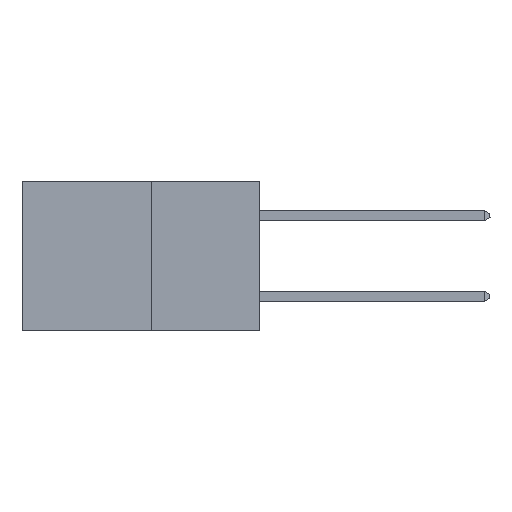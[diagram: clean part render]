
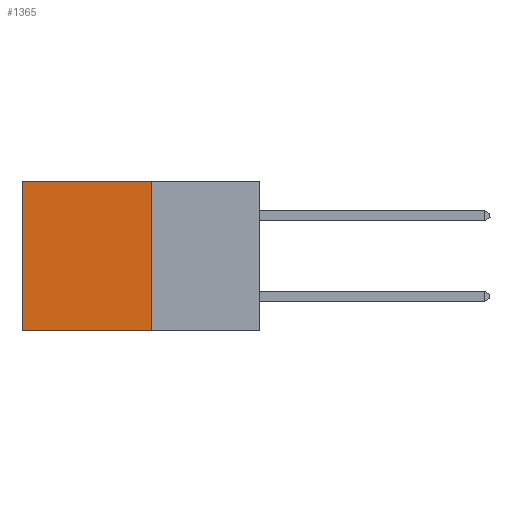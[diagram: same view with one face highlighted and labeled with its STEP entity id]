
A CAD part, left-side view. The second image highlights one B-rep face of the part: STEP entity #1365.
In plain terms, the highlighted planar face has unit normal (-1, 0, 0).
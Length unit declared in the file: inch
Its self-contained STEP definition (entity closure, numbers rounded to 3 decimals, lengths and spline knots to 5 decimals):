
#72 = EDGE_CURVE ( 'NONE', #12732, #971, #12079, .T. ) ;
#971 = VERTEX_POINT ( 'NONE', #7240 ) ;
#1365 = ADVANCED_FACE ( 'NONE', ( #10352 ), #4882, .F. ) ;
#2112 = EDGE_CURVE ( 'NONE', #16244, #12732, #8771, .T. ) ;
#2491 = ORIENTED_EDGE ( 'NONE', *, *, #5827, .F. ) ;
#3877 = VECTOR ( 'NONE', #14639, 39.37008 ) ;
#4882 = PLANE ( 'NONE',  #19514 ) ;
#5083 = CARTESIAN_POINT ( 'NONE',  ( 0.277, 0.59, 0. ) ) ;
#5406 = DIRECTION ( 'NONE',  ( 1., 0., 0. ) ) ;
#5827 = EDGE_CURVE ( 'NONE', #16244, #17717, #15740, .T. ) ;
#6088 = VECTOR ( 'NONE', #16671, 39.37008 ) ;
#6723 = ORIENTED_EDGE ( 'NONE', *, *, #2112, .T. ) ;
#6918 = DIRECTION ( 'NONE',  ( 0., 0., -1. ) ) ;
#7240 = CARTESIAN_POINT ( 'NONE',  ( 0.277, 0.59, -0.37 ) ) ;
#7446 = DIRECTION ( 'NONE',  ( 0., 0., -1. ) ) ;
#7618 = CARTESIAN_POINT ( 'NONE',  ( 0.277, 0.59, -0.37 ) ) ;
#8565 = EDGE_CURVE ( 'NONE', #17717, #971, #8808, .T. ) ;
#8771 = LINE ( 'NONE', #20213, #6088 ) ;
#8808 = LINE ( 'NONE', #16628, #3877 ) ;
#9876 = ORIENTED_EDGE ( 'NONE', *, *, #8565, .F. ) ;
#10352 = FACE_OUTER_BOUND ( 'NONE', #13102, .T. ) ;
#11012 = VECTOR ( 'NONE', #15985, 39.37008 ) ;
#12079 = LINE ( 'NONE', #7618, #15851 ) ;
#12732 = VERTEX_POINT ( 'NONE', #5083 ) ;
#13102 = EDGE_LOOP ( 'NONE', ( #19497, #9876, #2491, #6723 ) ) ;
#13620 = CARTESIAN_POINT ( 'NONE',  ( 0.277, 0.27, -0.37 ) ) ;
#14639 = DIRECTION ( 'NONE',  ( 0., 1., 0. ) ) ;
#15227 = CARTESIAN_POINT ( 'NONE',  ( 0.277, 0.27, -0.37 ) ) ;
#15740 = LINE ( 'NONE', #15227, #11012 ) ;
#15851 = VECTOR ( 'NONE', #7446, 39.37008 ) ;
#15985 = DIRECTION ( 'NONE',  ( 0., 0., -1. ) ) ;
#16244 = VERTEX_POINT ( 'NONE', #19821 ) ;
#16628 = CARTESIAN_POINT ( 'NONE',  ( 0.277, 0.27, -0.37 ) ) ;
#16671 = DIRECTION ( 'NONE',  ( 0., 1., 0. ) ) ;
#17717 = VERTEX_POINT ( 'NONE', #21259 ) ;
#19497 = ORIENTED_EDGE ( 'NONE', *, *, #72, .T. ) ;
#19514 = AXIS2_PLACEMENT_3D ( 'NONE', #13620, #5406, #6918 ) ;
#19821 = CARTESIAN_POINT ( 'NONE',  ( 0.277, 0.27, 0. ) ) ;
#20213 = CARTESIAN_POINT ( 'NONE',  ( 0.277, 0.27, 0. ) ) ;
#21259 = CARTESIAN_POINT ( 'NONE',  ( 0.277, 0.27, -0.37 ) ) ;
